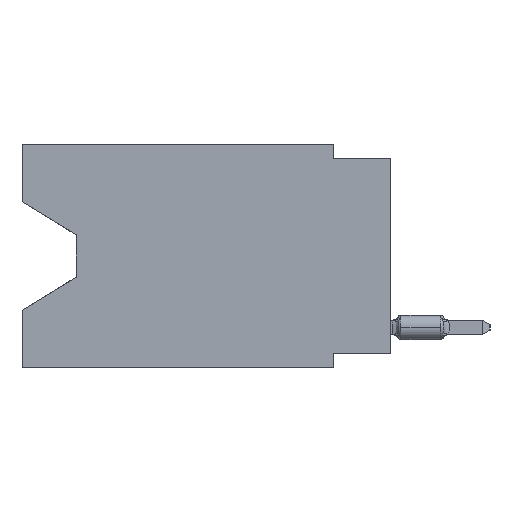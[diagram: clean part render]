
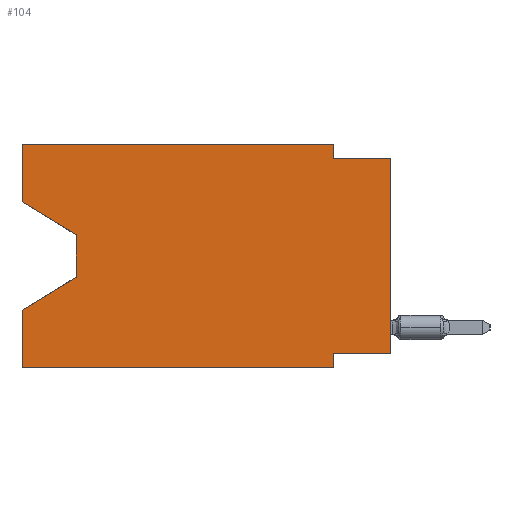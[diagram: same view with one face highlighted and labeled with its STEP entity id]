
A CAD part, left-side view. The second image highlights one B-rep face of the part: STEP entity #104.
In plain terms, the highlighted planar face has unit normal (-1, 0, 0).
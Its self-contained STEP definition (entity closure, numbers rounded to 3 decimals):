
#104 = ADVANCED_FACE ( 'NONE', ( #41804 ), #57558, .F. ) ;
#764 = EDGE_CURVE ( 'NONE', #9647, #36891, #59467, .T. ) ;
#2275 = CARTESIAN_POINT ( 'NONE',  ( 0., 16.383, 0. ) ) ;
#2501 = VERTEX_POINT ( 'NONE', #62953 ) ;
#3876 = CARTESIAN_POINT ( 'NONE',  ( 0., 16.383, -2.546 ) ) ;
#4650 = CARTESIAN_POINT ( 'NONE',  ( 0., 0., -0.635 ) ) ;
#4807 = VECTOR ( 'NONE', #18255, 1000. ) ;
#5531 = ORIENTED_EDGE ( 'NONE', *, *, #53582, .T. ) ;
#5635 = DIRECTION ( 'NONE',  ( 0., -1., 0. ) ) ;
#6856 = VERTEX_POINT ( 'NONE', #50562 ) ;
#8200 = VERTEX_POINT ( 'NONE', #8692 ) ;
#8222 = CARTESIAN_POINT ( 'NONE',  ( 0., 13.97, -4.013 ) ) ;
#8245 = EDGE_CURVE ( 'NONE', #56306, #2501, #41437, .T. ) ;
#8692 = CARTESIAN_POINT ( 'NONE',  ( 0., 16.383, -7.36 ) ) ;
#9647 = VERTEX_POINT ( 'NONE', #11482 ) ;
#10307 = ORIENTED_EDGE ( 'NONE', *, *, #56674, .F. ) ;
#11482 = CARTESIAN_POINT ( 'NONE',  ( 0., 16.383, -9.906 ) ) ;
#11709 = CARTESIAN_POINT ( 'NONE',  ( 0., 16.383, 0. ) ) ;
#11744 = EDGE_CURVE ( 'NONE', #16535, #46341, #13684, .T. ) ;
#11928 = VERTEX_POINT ( 'NONE', #61758 ) ;
#12627 = LINE ( 'NONE', #13279, #43005 ) ;
#12862 = LINE ( 'NONE', #48648, #52242 ) ;
#12904 = LINE ( 'NONE', #8222, #4807 ) ;
#13279 = CARTESIAN_POINT ( 'NONE',  ( 0., 13.97, -5.893 ) ) ;
#13550 = ORIENTED_EDGE ( 'NONE', *, *, #19447, .F. ) ;
#13684 = LINE ( 'NONE', #64569, #35953 ) ;
#13991 = VERTEX_POINT ( 'NONE', #16640 ) ;
#14869 = ORIENTED_EDGE ( 'NONE', *, *, #8245, .F. ) ;
#15601 = EDGE_CURVE ( 'NONE', #11928, #36891, #42939, .T. ) ;
#16223 = VECTOR ( 'NONE', #18960, 1000. ) ;
#16535 = VERTEX_POINT ( 'NONE', #3876 ) ;
#16640 = CARTESIAN_POINT ( 'NONE',  ( 0., 16.383, 0. ) ) ;
#17074 = DIRECTION ( 'NONE',  ( 0., 0., -1. ) ) ;
#17283 = EDGE_CURVE ( 'NONE', #16535, #13991, #48468, .T. ) ;
#17388 = DIRECTION ( 'NONE',  ( 0., 0., 1. ) ) ;
#18255 = DIRECTION ( 'NONE',  ( 0., 0., -1. ) ) ;
#18960 = DIRECTION ( 'NONE',  ( 0., -1., 0. ) ) ;
#19224 = CARTESIAN_POINT ( 'NONE',  ( 0., 2.54, -9.906 ) ) ;
#19447 = EDGE_CURVE ( 'NONE', #13991, #6856, #43203, .T. ) ;
#19965 = VECTOR ( 'NONE', #22526, 1000. ) ;
#21649 = CARTESIAN_POINT ( 'NONE',  ( 0., 13.97, -5.893 ) ) ;
#22368 = VERTEX_POINT ( 'NONE', #21649 ) ;
#22425 = EDGE_CURVE ( 'NONE', #22368, #8200, #12627, .T. ) ;
#22526 = DIRECTION ( 'NONE',  ( 0., 0., 1. ) ) ;
#26762 = DIRECTION ( 'NONE',  ( 0., 0., -1. ) ) ;
#27548 = CARTESIAN_POINT ( 'NONE',  ( 0., 0., 0. ) ) ;
#28139 = VECTOR ( 'NONE', #30101, 1000. ) ;
#28198 = LINE ( 'NONE', #27548, #19965 ) ;
#28200 = DIRECTION ( 'NONE',  ( 0., 0., -1. ) ) ;
#28976 = EDGE_CURVE ( 'NONE', #9647, #8200, #32731, .T. ) ;
#29952 = CARTESIAN_POINT ( 'NONE',  ( 0., 16.383, -9.906 ) ) ;
#30101 = DIRECTION ( 'NONE',  ( 0., -1., 0. ) ) ;
#32096 = DIRECTION ( 'NONE',  ( 1., 0., 0. ) ) ;
#32731 = LINE ( 'NONE', #2275, #56237 ) ;
#33083 = DIRECTION ( 'NONE',  ( 0., -0.855, -0.519 ) ) ;
#33300 = ORIENTED_EDGE ( 'NONE', *, *, #39099, .F. ) ;
#35953 = VECTOR ( 'NONE', #33083, 1000. ) ;
#36891 = VERTEX_POINT ( 'NONE', #19224 ) ;
#37013 = ORIENTED_EDGE ( 'NONE', *, *, #28976, .F. ) ;
#38107 = CARTESIAN_POINT ( 'NONE',  ( 0., 16.383, 0. ) ) ;
#39099 = EDGE_CURVE ( 'NONE', #6856, #56306, #47175, .T. ) ;
#39181 = ORIENTED_EDGE ( 'NONE', *, *, #15601, .F. ) ;
#40792 = ORIENTED_EDGE ( 'NONE', *, *, #11744, .T. ) ;
#41437 = LINE ( 'NONE', #4650, #56541 ) ;
#41804 = FACE_OUTER_BOUND ( 'NONE', #60233, .T. ) ;
#41848 = AXIS2_PLACEMENT_3D ( 'NONE', #11709, #32096, #17074 ) ;
#42939 = LINE ( 'NONE', #63390, #58805 ) ;
#43005 = VECTOR ( 'NONE', #48074, 1000. ) ;
#43203 = LINE ( 'NONE', #56224, #28139 ) ;
#44337 = EDGE_CURVE ( 'NONE', #46341, #22368, #12904, .T. ) ;
#44563 = ORIENTED_EDGE ( 'NONE', *, *, #17283, .F. ) ;
#44634 = DIRECTION ( 'NONE',  ( 0., 1., 0. ) ) ;
#45963 = ORIENTED_EDGE ( 'NONE', *, *, #22425, .T. ) ;
#46341 = VERTEX_POINT ( 'NONE', #54699 ) ;
#47175 = LINE ( 'NONE', #56250, #64371 ) ;
#48074 = DIRECTION ( 'NONE',  ( 0., 0.855, -0.519 ) ) ;
#48468 = LINE ( 'NONE', #38107, #49259 ) ;
#48648 = CARTESIAN_POINT ( 'NONE',  ( 0., 0., -9.271 ) ) ;
#48729 = CARTESIAN_POINT ( 'NONE',  ( 0., 2.54, -0.635 ) ) ;
#49259 = VECTOR ( 'NONE', #17388, 1000. ) ;
#50562 = CARTESIAN_POINT ( 'NONE',  ( 0., 2.54, 0. ) ) ;
#51301 = CARTESIAN_POINT ( 'NONE',  ( 0., 0., -9.271 ) ) ;
#52242 = VECTOR ( 'NONE', #44634, 1000. ) ;
#53582 = EDGE_CURVE ( 'NONE', #64610, #2501, #28198, .T. ) ;
#53789 = DIRECTION ( 'NONE',  ( 0., 0., 1. ) ) ;
#54699 = CARTESIAN_POINT ( 'NONE',  ( 0., 13.97, -4.013 ) ) ;
#56224 = CARTESIAN_POINT ( 'NONE',  ( 0., 16.383, 0. ) ) ;
#56237 = VECTOR ( 'NONE', #53789, 1000. ) ;
#56250 = CARTESIAN_POINT ( 'NONE',  ( 0., 2.54, 0. ) ) ;
#56306 = VERTEX_POINT ( 'NONE', #48729 ) ;
#56541 = VECTOR ( 'NONE', #5635, 1000. ) ;
#56674 = EDGE_CURVE ( 'NONE', #64610, #11928, #12862, .T. ) ;
#57558 = PLANE ( 'NONE',  #41848 ) ;
#58805 = VECTOR ( 'NONE', #28200, 1000. ) ;
#59467 = LINE ( 'NONE', #29952, #16223 ) ;
#60233 = EDGE_LOOP ( 'NONE', ( #40792, #64671, #45963, #37013, #63842, #39181, #10307, #5531, #14869, #33300, #13550, #44563 ) ) ;
#61758 = CARTESIAN_POINT ( 'NONE',  ( 0., 2.54, -9.271 ) ) ;
#62953 = CARTESIAN_POINT ( 'NONE',  ( 0., 0., -0.635 ) ) ;
#63390 = CARTESIAN_POINT ( 'NONE',  ( 0., 2.54, -9.906 ) ) ;
#63842 = ORIENTED_EDGE ( 'NONE', *, *, #764, .T. ) ;
#64371 = VECTOR ( 'NONE', #26762, 1000. ) ;
#64569 = CARTESIAN_POINT ( 'NONE',  ( 0., 16.383, -2.546 ) ) ;
#64610 = VERTEX_POINT ( 'NONE', #51301 ) ;
#64671 = ORIENTED_EDGE ( 'NONE', *, *, #44337, .T. ) ;
